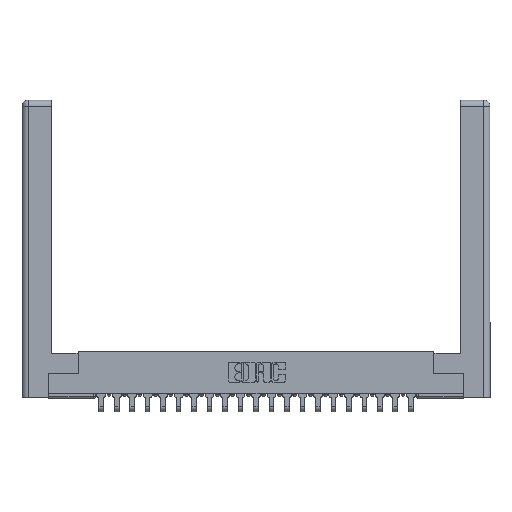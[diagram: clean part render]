
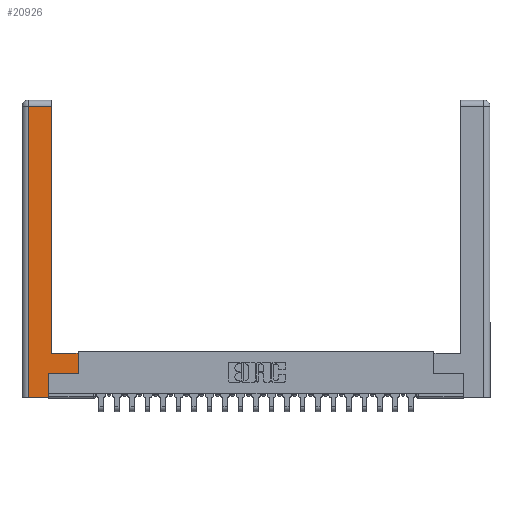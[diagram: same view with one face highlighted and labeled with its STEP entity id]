
A CAD part, top view. The second image highlights one B-rep face of the part: STEP entity #20926.
In plain terms, the highlighted planar face has unit normal (0, 0, 1).
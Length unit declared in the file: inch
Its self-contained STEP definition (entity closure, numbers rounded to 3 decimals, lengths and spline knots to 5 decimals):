
#177 = VERTEX_POINT ( 'NONE', #10948 ) ;
#810 = EDGE_CURVE ( 'NONE', #177, #15948, #4778, .T. ) ;
#851 = CARTESIAN_POINT ( 'NONE',  ( 0.565, 0.45, 0. ) ) ;
#1070 = CARTESIAN_POINT ( 'NONE',  ( 0.265, 0., 0. ) ) ;
#1548 = CARTESIAN_POINT ( 'NONE',  ( 0.0615, 0., 0. ) ) ;
#1561 = CARTESIAN_POINT ( 'NONE',  ( 0.295, 3., 0. ) ) ;
#1730 = EDGE_CURVE ( 'NONE', #4993, #17547, #1902, .T. ) ;
#1902 = LINE ( 'NONE', #15860, #14573 ) ;
#2544 = CARTESIAN_POINT ( 'NONE',  ( 0.295, 0.45, 0. ) ) ;
#3480 = LINE ( 'NONE', #14350, #18384 ) ;
#3488 = ORIENTED_EDGE ( 'NONE', *, *, #15421, .T. ) ;
#4007 = VERTEX_POINT ( 'NONE', #2544 ) ;
#4056 = LINE ( 'NONE', #9260, #13622 ) ;
#4594 = ORIENTED_EDGE ( 'NONE', *, *, #1730, .T. ) ;
#4778 = LINE ( 'NONE', #12595, #18547 ) ;
#4849 = VECTOR ( 'NONE', #17690, 39.37008 ) ;
#4993 = VERTEX_POINT ( 'NONE', #1070 ) ;
#5383 = DIRECTION ( 'NONE',  ( -1., 0., 0. ) ) ;
#5783 = ORIENTED_EDGE ( 'NONE', *, *, #8079, .T. ) ;
#6367 = ORIENTED_EDGE ( 'NONE', *, *, #18546, .T. ) ;
#6856 = PLANE ( 'NONE',  #15506 ) ;
#7039 = DIRECTION ( 'NONE',  ( 1., 0., 0. ) ) ;
#7389 = ORIENTED_EDGE ( 'NONE', *, *, #810, .T. ) ;
#7479 = DIRECTION ( 'NONE',  ( -1., 0., 0. ) ) ;
#7486 = EDGE_CURVE ( 'NONE', #22380, #4007, #21214, .T. ) ;
#7583 = EDGE_CURVE ( 'NONE', #17547, #11467, #3480, .T. ) ;
#8079 = EDGE_CURVE ( 'NONE', #21452, #4993, #20940, .T. ) ;
#8388 = DIRECTION ( 'NONE',  ( 0., 1., 0. ) ) ;
#8796 = DIRECTION ( 'NONE',  ( 0., 1., 0. ) ) ;
#9260 = CARTESIAN_POINT ( 'NONE',  ( 0.0615, 0., 0. ) ) ;
#9513 = LINE ( 'NONE', #15964, #14300 ) ;
#9624 = LINE ( 'NONE', #1561, #4849 ) ;
#9729 = DIRECTION ( 'NONE',  ( 0., -1., 0. ) ) ;
#10758 = ORIENTED_EDGE ( 'NONE', *, *, #7583, .T. ) ;
#10948 = CARTESIAN_POINT ( 'NONE',  ( 0.295, 2.94, 0. ) ) ;
#11467 = VERTEX_POINT ( 'NONE', #16320 ) ;
#12595 = CARTESIAN_POINT ( 'NONE',  ( 0.0615, 2.94, 0. ) ) ;
#13622 = VECTOR ( 'NONE', #9729, 39.37008 ) ;
#14110 = ORIENTED_EDGE ( 'NONE', *, *, #16659, .T. ) ;
#14151 = DIRECTION ( 'NONE',  ( -1., 0., 0. ) ) ;
#14300 = VECTOR ( 'NONE', #8796, 39.37008 ) ;
#14350 = CARTESIAN_POINT ( 'NONE',  ( 0.565, 0.245, 0. ) ) ;
#14540 = CARTESIAN_POINT ( 'NONE',  ( 0.295, 0.45, 0. ) ) ;
#14573 = VECTOR ( 'NONE', #8388, 39.37008 ) ;
#14888 = EDGE_LOOP ( 'NONE', ( #14110, #7389, #3488, #5783, #4594, #10758, #6367, #16673 ) ) ;
#14891 = CARTESIAN_POINT ( 'NONE',  ( 0.265, 0.245, 0. ) ) ;
#15280 = VECTOR ( 'NONE', #18855, 39.37008 ) ;
#15421 = EDGE_CURVE ( 'NONE', #15948, #21452, #4056, .T. ) ;
#15506 = AXIS2_PLACEMENT_3D ( 'NONE', #21175, #21256, #14151 ) ;
#15564 = VECTOR ( 'NONE', #7479, 39.37008 ) ;
#15860 = CARTESIAN_POINT ( 'NONE',  ( 0.265, 0.245, 0. ) ) ;
#15948 = VERTEX_POINT ( 'NONE', #16788 ) ;
#15964 = CARTESIAN_POINT ( 'NONE',  ( 0.565, 0.45, 0. ) ) ;
#16320 = CARTESIAN_POINT ( 'NONE',  ( 0.565, 0.245, 0. ) ) ;
#16659 = EDGE_CURVE ( 'NONE', #4007, #177, #9624, .T. ) ;
#16673 = ORIENTED_EDGE ( 'NONE', *, *, #7486, .T. ) ;
#16788 = CARTESIAN_POINT ( 'NONE',  ( 0.0615, 2.94, 0. ) ) ;
#17206 = CARTESIAN_POINT ( 'NONE',  ( 0.265, 0., 0. ) ) ;
#17547 = VERTEX_POINT ( 'NONE', #14891 ) ;
#17690 = DIRECTION ( 'NONE',  ( 0., 1., 0. ) ) ;
#18384 = VECTOR ( 'NONE', #7039, 39.37008 ) ;
#18546 = EDGE_CURVE ( 'NONE', #11467, #22380, #9513, .T. ) ;
#18547 = VECTOR ( 'NONE', #5383, 39.37008 ) ;
#18855 = DIRECTION ( 'NONE',  ( 1., 0., 0. ) ) ;
#20926 = ADVANCED_FACE ( 'NONE', ( #22809 ), #6856, .F. ) ;
#20940 = LINE ( 'NONE', #17206, #15280 ) ;
#21175 = CARTESIAN_POINT ( 'NONE',  ( 0., 0., 0. ) ) ;
#21214 = LINE ( 'NONE', #14540, #15564 ) ;
#21256 = DIRECTION ( 'NONE',  ( 0., 0., -1. ) ) ;
#21452 = VERTEX_POINT ( 'NONE', #1548 ) ;
#22380 = VERTEX_POINT ( 'NONE', #851 ) ;
#22809 = FACE_OUTER_BOUND ( 'NONE', #14888, .T. ) ;
